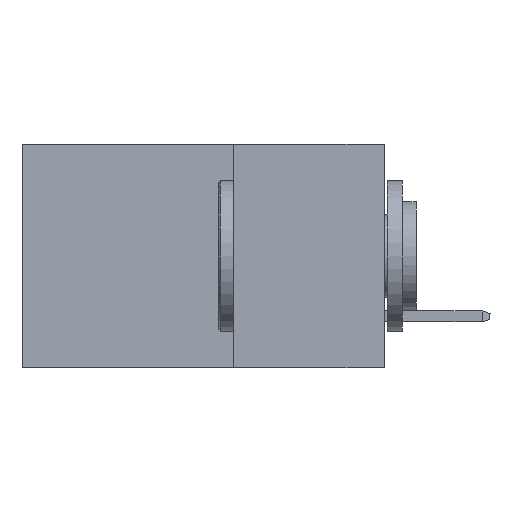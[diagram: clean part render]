
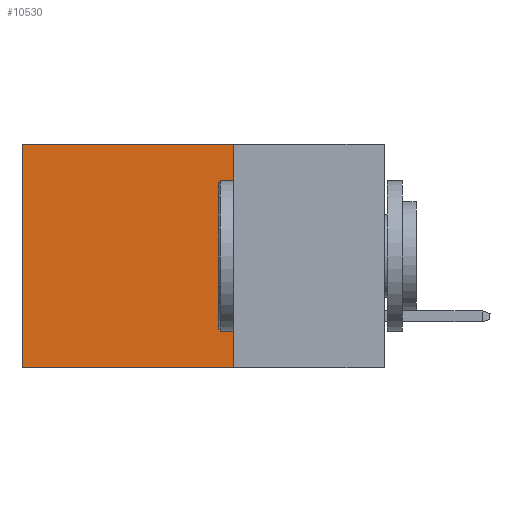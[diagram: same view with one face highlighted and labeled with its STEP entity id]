
A CAD part, left-side view. The second image highlights one B-rep face of the part: STEP entity #10530.
In plain terms, the highlighted planar face has unit normal (-1, 0, 0).
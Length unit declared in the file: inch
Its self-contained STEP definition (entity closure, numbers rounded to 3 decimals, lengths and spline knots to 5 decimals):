
#827 = EDGE_CURVE ( 'NONE', #4935, #9555, #4040, .T. ) ;
#1541 = CARTESIAN_POINT ( 'NONE',  ( 0.2615, 0.6, 0. ) ) ;
#1688 = FACE_OUTER_BOUND ( 'NONE', #5066, .T. ) ;
#1720 = VECTOR ( 'NONE', #3090, 39.37008 ) ;
#1756 = LINE ( 'NONE', #5607, #5497 ) ;
#2641 = DIRECTION ( 'NONE',  ( 1., 0., 0. ) ) ;
#2765 = PLANE ( 'NONE',  #7478 ) ;
#2766 = ORIENTED_EDGE ( 'NONE', *, *, #5878, .F. ) ;
#3090 = DIRECTION ( 'NONE',  ( 0., 1., 0. ) ) ;
#3235 = VERTEX_POINT ( 'NONE', #8185 ) ;
#3653 = DIRECTION ( 'NONE',  ( 0., 0., -1. ) ) ;
#4040 = LINE ( 'NONE', #7929, #1720 ) ;
#4228 = VERTEX_POINT ( 'NONE', #1541 ) ;
#4935 = VERTEX_POINT ( 'NONE', #7228 ) ;
#5039 = VECTOR ( 'NONE', #7836, 39.37008 ) ;
#5066 = EDGE_LOOP ( 'NONE', ( #9282, #11083, #2766, #7992 ) ) ;
#5198 = CARTESIAN_POINT ( 'NONE',  ( 0.2615, 0.25, -0.37 ) ) ;
#5497 = VECTOR ( 'NONE', #12328, 39.37008 ) ;
#5607 = CARTESIAN_POINT ( 'NONE',  ( 0.2615, 0.6, -0.37 ) ) ;
#5751 = EDGE_CURVE ( 'NONE', #3235, #4228, #7719, .T. ) ;
#5878 = EDGE_CURVE ( 'NONE', #3235, #4935, #9913, .T. ) ;
#7228 = CARTESIAN_POINT ( 'NONE',  ( 0.2615, 0.25, -0.37 ) ) ;
#7478 = AXIS2_PLACEMENT_3D ( 'NONE', #9384, #2641, #3653 ) ;
#7719 = LINE ( 'NONE', #11555, #5039 ) ;
#7836 = DIRECTION ( 'NONE',  ( 0., 1., 0. ) ) ;
#7929 = CARTESIAN_POINT ( 'NONE',  ( 0.2615, 0.25, -0.37 ) ) ;
#7992 = ORIENTED_EDGE ( 'NONE', *, *, #5751, .T. ) ;
#8185 = CARTESIAN_POINT ( 'NONE',  ( 0.2615, 0.25, 0. ) ) ;
#9282 = ORIENTED_EDGE ( 'NONE', *, *, #10553, .T. ) ;
#9384 = CARTESIAN_POINT ( 'NONE',  ( 0.2615, 0.25, -0.37 ) ) ;
#9555 = VERTEX_POINT ( 'NONE', #12323 ) ;
#9653 = VECTOR ( 'NONE', #11791, 39.37008 ) ;
#9913 = LINE ( 'NONE', #5198, #9653 ) ;
#10530 = ADVANCED_FACE ( 'NONE', ( #1688 ), #2765, .F. ) ;
#10553 = EDGE_CURVE ( 'NONE', #4228, #9555, #1756, .T. ) ;
#11083 = ORIENTED_EDGE ( 'NONE', *, *, #827, .F. ) ;
#11555 = CARTESIAN_POINT ( 'NONE',  ( 0.2615, 0.25, 0. ) ) ;
#11791 = DIRECTION ( 'NONE',  ( 0., 0., -1. ) ) ;
#12323 = CARTESIAN_POINT ( 'NONE',  ( 0.2615, 0.6, -0.37 ) ) ;
#12328 = DIRECTION ( 'NONE',  ( 0., 0., -1. ) ) ;
